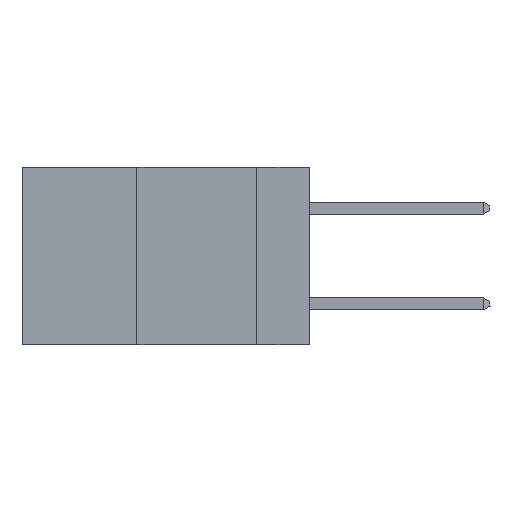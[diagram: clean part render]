
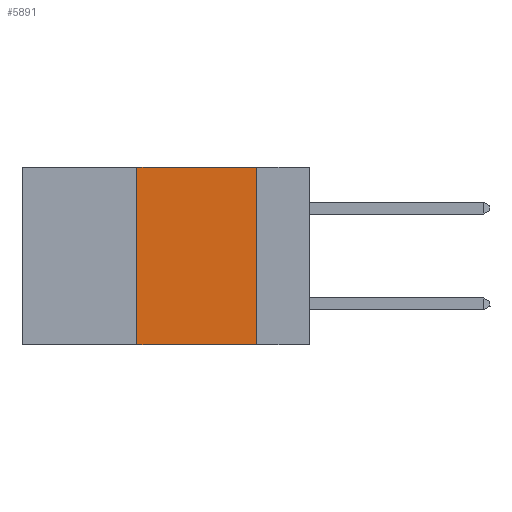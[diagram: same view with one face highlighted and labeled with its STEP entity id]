
A CAD part, left-side view. The second image highlights one B-rep face of the part: STEP entity #5891.
In plain terms, the highlighted planar face has unit normal (-1, 0, 0).
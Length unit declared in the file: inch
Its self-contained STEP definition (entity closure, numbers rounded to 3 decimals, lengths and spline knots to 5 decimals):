
#537 = AXIS2_PLACEMENT_3D ( 'NONE', #984, #29556, #10667 ) ;
#984 = CARTESIAN_POINT ( 'NONE',  ( 0., 0.6, 0. ) ) ;
#1848 = ORIENTED_EDGE ( 'NONE', *, *, #40860, .F. ) ;
#1942 = VERTEX_POINT ( 'NONE', #25221 ) ;
#2672 = CARTESIAN_POINT ( 'NONE',  ( 0., 0.36, 0. ) ) ;
#5891 = ADVANCED_FACE ( 'NONE', ( #22886 ), #7464, .F. ) ;
#7464 = PLANE ( 'NONE',  #537 ) ;
#10667 = DIRECTION ( 'NONE',  ( 0., 0., -1. ) ) ;
#10977 = CARTESIAN_POINT ( 'NONE',  ( 0., 0.6, -0.37 ) ) ;
#11063 = CARTESIAN_POINT ( 'NONE',  ( 0., 0.11, 0. ) ) ;
#11191 = CARTESIAN_POINT ( 'NONE',  ( 0., 0.6, 0. ) ) ;
#13261 = VERTEX_POINT ( 'NONE', #15455 ) ;
#14170 = DIRECTION ( 'NONE',  ( 0., -1., 0. ) ) ;
#14745 = LINE ( 'NONE', #10977, #23146 ) ;
#15029 = CARTESIAN_POINT ( 'NONE',  ( 0., 0.11, 0. ) ) ;
#15292 = LINE ( 'NONE', #11191, #32013 ) ;
#15345 = ORIENTED_EDGE ( 'NONE', *, *, #29774, .F. ) ;
#15371 = DIRECTION ( 'NONE',  ( 0., 0., 1. ) ) ;
#15455 = CARTESIAN_POINT ( 'NONE',  ( 0., 0.11, -0.37 ) ) ;
#15811 = VERTEX_POINT ( 'NONE', #37138 ) ;
#19602 = LINE ( 'NONE', #2672, #36303 ) ;
#22059 = EDGE_LOOP ( 'NONE', ( #1848, #15345, #38509, #29280 ) ) ;
#22886 = FACE_OUTER_BOUND ( 'NONE', #22059, .T. ) ;
#23146 = VECTOR ( 'NONE', #14170, 39.37008 ) ;
#23796 = EDGE_CURVE ( 'NONE', #15811, #1942, #19602, .T. ) ;
#24083 = LINE ( 'NONE', #15029, #31416 ) ;
#25221 = CARTESIAN_POINT ( 'NONE',  ( 0., 0.36, 0. ) ) ;
#29280 = ORIENTED_EDGE ( 'NONE', *, *, #38225, .T. ) ;
#29556 = DIRECTION ( 'NONE',  ( 1., 0., 0. ) ) ;
#29774 = EDGE_CURVE ( 'NONE', #1942, #36625, #15292, .T. ) ;
#30073 = DIRECTION ( 'NONE',  ( 0., -1., 0. ) ) ;
#30861 = DIRECTION ( 'NONE',  ( 0., 0., -1. ) ) ;
#31416 = VECTOR ( 'NONE', #30861, 39.37008 ) ;
#32013 = VECTOR ( 'NONE', #30073, 39.37008 ) ;
#36303 = VECTOR ( 'NONE', #15371, 39.37008 ) ;
#36625 = VERTEX_POINT ( 'NONE', #11063 ) ;
#37138 = CARTESIAN_POINT ( 'NONE',  ( 0., 0.36, -0.37 ) ) ;
#38225 = EDGE_CURVE ( 'NONE', #15811, #13261, #14745, .T. ) ;
#38509 = ORIENTED_EDGE ( 'NONE', *, *, #23796, .F. ) ;
#40860 = EDGE_CURVE ( 'NONE', #36625, #13261, #24083, .T. ) ;
